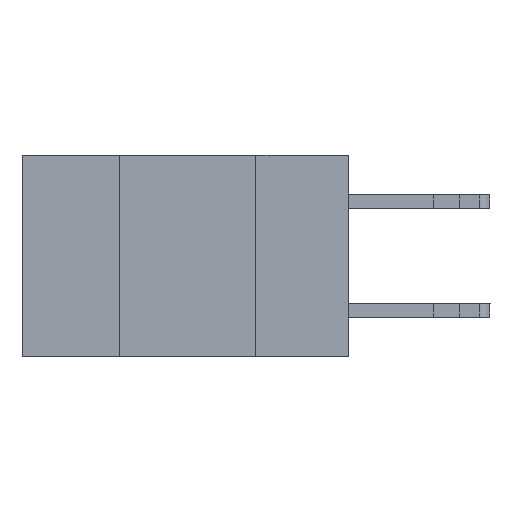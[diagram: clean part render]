
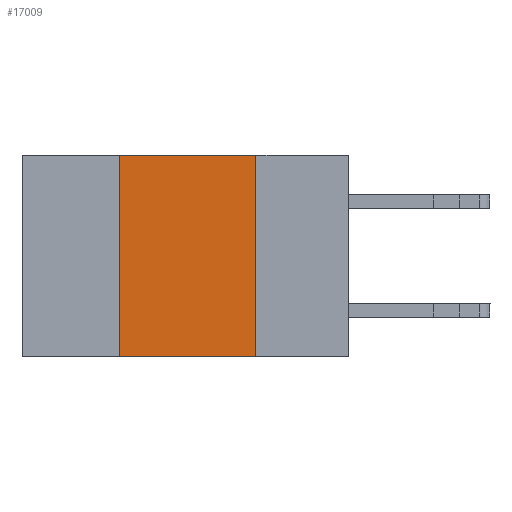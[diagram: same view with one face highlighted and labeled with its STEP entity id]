
A CAD part, left-side view. The second image highlights one B-rep face of the part: STEP entity #17009.
In plain terms, the highlighted planar face has unit normal (-1, 0, 0).
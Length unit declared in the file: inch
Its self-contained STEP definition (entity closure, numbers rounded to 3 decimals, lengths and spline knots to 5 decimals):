
#279 = DIRECTION ( 'NONE',  ( 0., 0., 1. ) ) ;
#1833 = FACE_OUTER_BOUND ( 'NONE', #9945, .T. ) ;
#1862 = CARTESIAN_POINT ( 'NONE',  ( 0., 0.42, 0. ) ) ;
#2029 = CARTESIAN_POINT ( 'NONE',  ( 0., 0.6, -0.37 ) ) ;
#2044 = EDGE_CURVE ( 'NONE', #5578, #5678, #9082, .T. ) ;
#3467 = DIRECTION ( 'NONE',  ( 0., -1., 0. ) ) ;
#4287 = ORIENTED_EDGE ( 'NONE', *, *, #12525, .T. ) ;
#4419 = ORIENTED_EDGE ( 'NONE', *, *, #2044, .F. ) ;
#4535 = CARTESIAN_POINT ( 'NONE',  ( 0., 0.6, 0. ) ) ;
#5488 = VERTEX_POINT ( 'NONE', #6684 ) ;
#5537 = DIRECTION ( 'NONE',  ( 0., 0., -1. ) ) ;
#5578 = VERTEX_POINT ( 'NONE', #13540 ) ;
#5678 = VERTEX_POINT ( 'NONE', #1862 ) ;
#6670 = AXIS2_PLACEMENT_3D ( 'NONE', #15703, #8946, #15527 ) ;
#6684 = CARTESIAN_POINT ( 'NONE',  ( 0., 0.17, -0.37 ) ) ;
#6880 = VECTOR ( 'NONE', #5537, 39.37008 ) ;
#7133 = DIRECTION ( 'NONE',  ( 0., -1., 0. ) ) ;
#7170 = LINE ( 'NONE', #2029, #13347 ) ;
#8946 = DIRECTION ( 'NONE',  ( 1., 0., 0. ) ) ;
#9066 = VECTOR ( 'NONE', #3467, 39.37008 ) ;
#9082 = LINE ( 'NONE', #14687, #14494 ) ;
#9480 = CARTESIAN_POINT ( 'NONE',  ( 0., 0.17, 0. ) ) ;
#9543 = CARTESIAN_POINT ( 'NONE',  ( 0., 0.17, 0. ) ) ;
#9945 = EDGE_LOOP ( 'NONE', ( #11499, #14551, #4419, #4287 ) ) ;
#10122 = LINE ( 'NONE', #9543, #6880 ) ;
#11499 = ORIENTED_EDGE ( 'NONE', *, *, #14430, .F. ) ;
#12525 = EDGE_CURVE ( 'NONE', #5578, #5488, #7170, .T. ) ;
#12960 = PLANE ( 'NONE',  #6670 ) ;
#13347 = VECTOR ( 'NONE', #7133, 39.37008 ) ;
#13540 = CARTESIAN_POINT ( 'NONE',  ( 0., 0.42, -0.37 ) ) ;
#14430 = EDGE_CURVE ( 'NONE', #16710, #5488, #10122, .T. ) ;
#14494 = VECTOR ( 'NONE', #279, 39.37008 ) ;
#14551 = ORIENTED_EDGE ( 'NONE', *, *, #16125, .F. ) ;
#14687 = CARTESIAN_POINT ( 'NONE',  ( 0., 0.42, 0. ) ) ;
#15527 = DIRECTION ( 'NONE',  ( 0., 0., -1. ) ) ;
#15703 = CARTESIAN_POINT ( 'NONE',  ( 0., 0.6, 0. ) ) ;
#15952 = LINE ( 'NONE', #4535, #9066 ) ;
#16125 = EDGE_CURVE ( 'NONE', #5678, #16710, #15952, .T. ) ;
#16710 = VERTEX_POINT ( 'NONE', #9480 ) ;
#17009 = ADVANCED_FACE ( 'NONE', ( #1833 ), #12960, .F. ) ;
